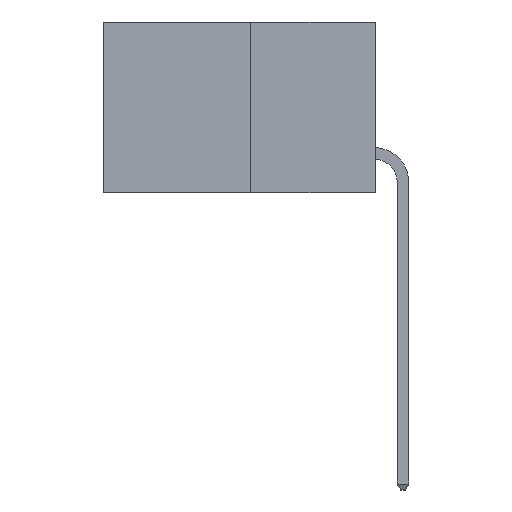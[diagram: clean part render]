
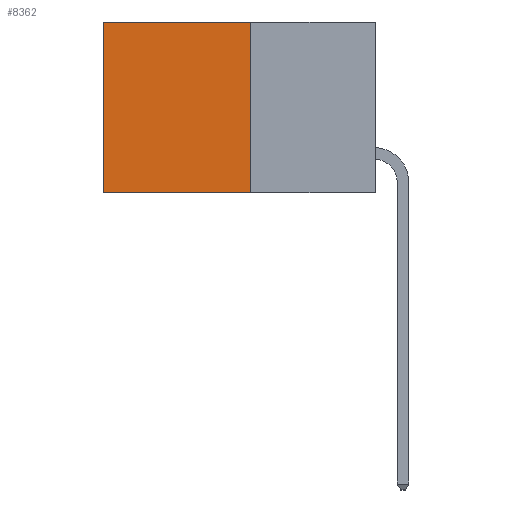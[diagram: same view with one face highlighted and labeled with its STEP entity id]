
A CAD part, left-side view. The second image highlights one B-rep face of the part: STEP entity #8362.
In plain terms, the highlighted planar face has unit normal (-1, 0, 0).
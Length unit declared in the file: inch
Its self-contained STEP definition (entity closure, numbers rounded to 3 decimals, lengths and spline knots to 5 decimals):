
#72 = DIRECTION ( 'NONE',  ( 0., 1., 0. ) ) ;
#207 = CARTESIAN_POINT ( 'NONE',  ( 0.277, 0.27, -0.37 ) ) ;
#815 = ORIENTED_EDGE ( 'NONE', *, *, #2817, .T. ) ;
#948 = DIRECTION ( 'NONE',  ( 0., 1., 0. ) ) ;
#1256 = VERTEX_POINT ( 'NONE', #1760 ) ;
#1519 = AXIS2_PLACEMENT_3D ( 'NONE', #2494, #2492, #2479 ) ;
#1760 = CARTESIAN_POINT ( 'NONE',  ( 0.277, 0.27, 0. ) ) ;
#2026 = ORIENTED_EDGE ( 'NONE', *, *, #13723, .F. ) ;
#2168 = EDGE_CURVE ( 'NONE', #6929, #3517, #13181, .T. ) ;
#2175 = FACE_OUTER_BOUND ( 'NONE', #3931, .T. ) ;
#2479 = DIRECTION ( 'NONE',  ( 0., 0., -1. ) ) ;
#2492 = DIRECTION ( 'NONE',  ( 1., 0., 0. ) ) ;
#2494 = CARTESIAN_POINT ( 'NONE',  ( 0.277, 0.27, -0.37 ) ) ;
#2502 = VECTOR ( 'NONE', #72, 39.37008 ) ;
#2643 = PLANE ( 'NONE',  #1519 ) ;
#2755 = EDGE_CURVE ( 'NONE', #3793, #3517, #8265, .T. ) ;
#2817 = EDGE_CURVE ( 'NONE', #1256, #6929, #12660, .T. ) ;
#2953 = DIRECTION ( 'NONE',  ( 0., 0., -1. ) ) ;
#2965 = ORIENTED_EDGE ( 'NONE', *, *, #2755, .F. ) ;
#3517 = VERTEX_POINT ( 'NONE', #9245 ) ;
#3793 = VERTEX_POINT ( 'NONE', #6057 ) ;
#3931 = EDGE_LOOP ( 'NONE', ( #7119, #2965, #2026, #815 ) ) ;
#6057 = CARTESIAN_POINT ( 'NONE',  ( 0.277, 0.27, -0.37 ) ) ;
#6929 = VERTEX_POINT ( 'NONE', #13658 ) ;
#7119 = ORIENTED_EDGE ( 'NONE', *, *, #2168, .T. ) ;
#7327 = CARTESIAN_POINT ( 'NONE',  ( 0.277, 0.27, -0.37 ) ) ;
#7486 = VECTOR ( 'NONE', #2953, 39.37008 ) ;
#7632 = VECTOR ( 'NONE', #948, 39.37008 ) ;
#7799 = LINE ( 'NONE', #7327, #7486 ) ;
#7999 = DIRECTION ( 'NONE',  ( 0., 0., -1. ) ) ;
#8265 = LINE ( 'NONE', #207, #2502 ) ;
#8362 = ADVANCED_FACE ( 'NONE', ( #2175 ), #2643, .F. ) ;
#8489 = CARTESIAN_POINT ( 'NONE',  ( 0.277, 0.59, -0.37 ) ) ;
#9090 = CARTESIAN_POINT ( 'NONE',  ( 0.277, 0.27, 0. ) ) ;
#9245 = CARTESIAN_POINT ( 'NONE',  ( 0.277, 0.59, -0.37 ) ) ;
#12207 = VECTOR ( 'NONE', #7999, 39.37008 ) ;
#12660 = LINE ( 'NONE', #9090, #7632 ) ;
#13181 = LINE ( 'NONE', #8489, #12207 ) ;
#13658 = CARTESIAN_POINT ( 'NONE',  ( 0.277, 0.59, 0. ) ) ;
#13723 = EDGE_CURVE ( 'NONE', #1256, #3793, #7799, .T. ) ;
